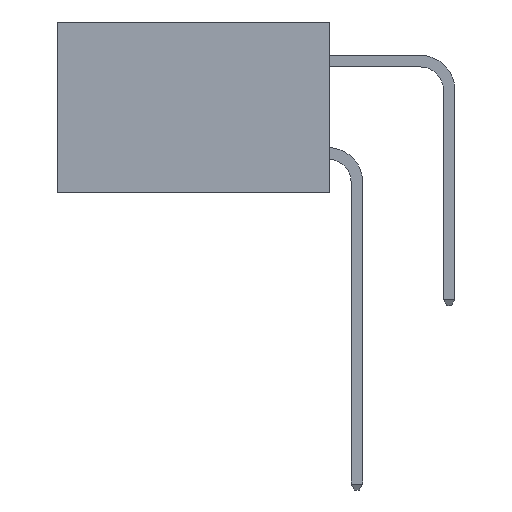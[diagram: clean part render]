
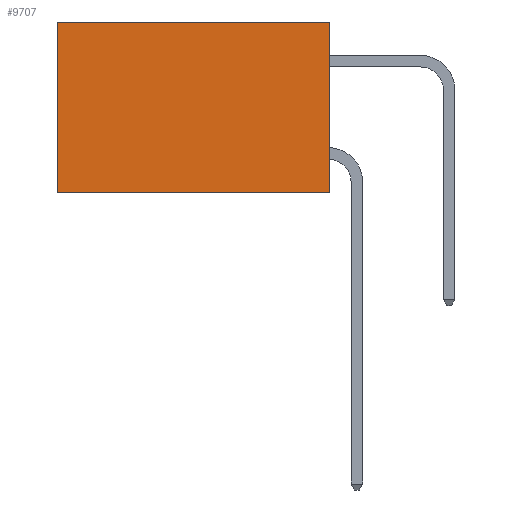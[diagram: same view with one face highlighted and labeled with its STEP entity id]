
A CAD part, left-side view. The second image highlights one B-rep face of the part: STEP entity #9707.
In plain terms, the highlighted planar face has unit normal (-1, 0, 0).
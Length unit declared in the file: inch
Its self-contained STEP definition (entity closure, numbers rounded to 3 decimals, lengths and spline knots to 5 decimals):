
#172 = CARTESIAN_POINT ( 'NONE',  ( 0.277, 0., -0.37 ) ) ;
#311 = VERTEX_POINT ( 'NONE', #1392 ) ;
#1089 = LINE ( 'NONE', #13438, #12182 ) ;
#1392 = CARTESIAN_POINT ( 'NONE',  ( 0.277, 0.59, 0. ) ) ;
#2042 = EDGE_CURVE ( 'NONE', #311, #18207, #3847, .T. ) ;
#2105 = VERTEX_POINT ( 'NONE', #16393 ) ;
#2679 = VECTOR ( 'NONE', #18490, 39.37008 ) ;
#3117 = LINE ( 'NONE', #7678, #2679 ) ;
#3269 = DIRECTION ( 'NONE',  ( 0., 1., 0. ) ) ;
#3456 = EDGE_CURVE ( 'NONE', #2105, #311, #3117, .T. ) ;
#3842 = LINE ( 'NONE', #9270, #11098 ) ;
#3847 = LINE ( 'NONE', #16852, #18291 ) ;
#4292 = DIRECTION ( 'NONE',  ( 0., 0., -1. ) ) ;
#5990 = PLANE ( 'NONE',  #12891 ) ;
#6619 = CARTESIAN_POINT ( 'NONE',  ( 0.277, 0., -0.37 ) ) ;
#7275 = FACE_OUTER_BOUND ( 'NONE', #17364, .T. ) ;
#7504 = DIRECTION ( 'NONE',  ( 0., 0., -1. ) ) ;
#7678 = CARTESIAN_POINT ( 'NONE',  ( 0.277, 0., 0. ) ) ;
#7889 = DIRECTION ( 'NONE',  ( 0., 0., -1. ) ) ;
#8213 = ORIENTED_EDGE ( 'NONE', *, *, #9230, .F. ) ;
#9230 = EDGE_CURVE ( 'NONE', #2105, #12858, #3842, .T. ) ;
#9270 = CARTESIAN_POINT ( 'NONE',  ( 0.277, 0., -0.37 ) ) ;
#9590 = ORIENTED_EDGE ( 'NONE', *, *, #2042, .T. ) ;
#9707 = ADVANCED_FACE ( 'NONE', ( #7275 ), #5990, .F. ) ;
#9750 = ORIENTED_EDGE ( 'NONE', *, *, #10780, .F. ) ;
#10780 = EDGE_CURVE ( 'NONE', #12858, #18207, #1089, .T. ) ;
#11098 = VECTOR ( 'NONE', #7889, 39.37008 ) ;
#12182 = VECTOR ( 'NONE', #3269, 39.37008 ) ;
#12529 = ORIENTED_EDGE ( 'NONE', *, *, #3456, .T. ) ;
#12858 = VERTEX_POINT ( 'NONE', #6619 ) ;
#12891 = AXIS2_PLACEMENT_3D ( 'NONE', #172, #16105, #7504 ) ;
#13438 = CARTESIAN_POINT ( 'NONE',  ( 0.277, 0., -0.37 ) ) ;
#16105 = DIRECTION ( 'NONE',  ( 1., 0., 0. ) ) ;
#16122 = CARTESIAN_POINT ( 'NONE',  ( 0.277, 0.59, -0.37 ) ) ;
#16393 = CARTESIAN_POINT ( 'NONE',  ( 0.277, 0., 0. ) ) ;
#16852 = CARTESIAN_POINT ( 'NONE',  ( 0.277, 0.59, -0.37 ) ) ;
#17364 = EDGE_LOOP ( 'NONE', ( #9590, #9750, #8213, #12529 ) ) ;
#18207 = VERTEX_POINT ( 'NONE', #16122 ) ;
#18291 = VECTOR ( 'NONE', #4292, 39.37008 ) ;
#18490 = DIRECTION ( 'NONE',  ( 0., 1., 0. ) ) ;
